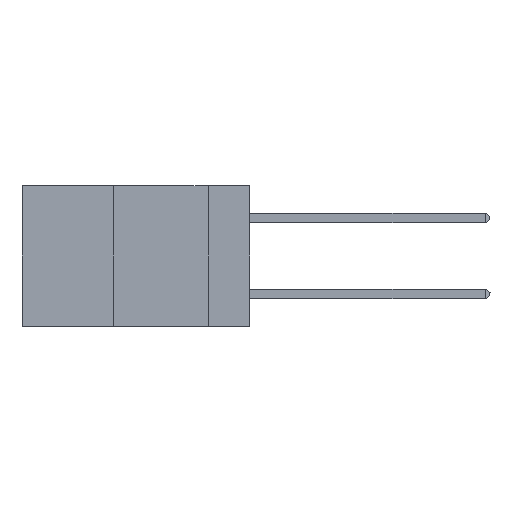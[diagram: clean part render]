
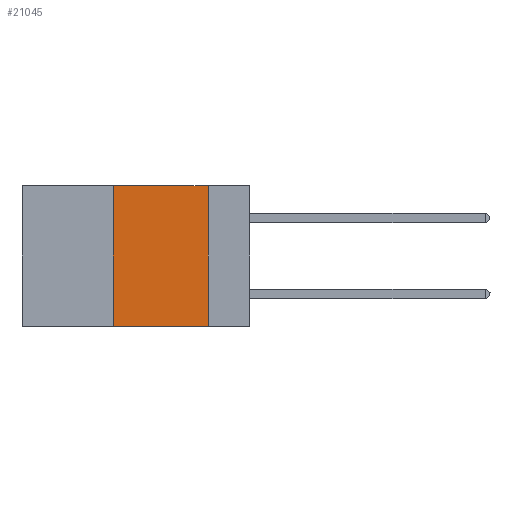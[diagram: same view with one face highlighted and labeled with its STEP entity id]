
A CAD part, left-side view. The second image highlights one B-rep face of the part: STEP entity #21045.
In plain terms, the highlighted planar face has unit normal (-1, 0, 0).
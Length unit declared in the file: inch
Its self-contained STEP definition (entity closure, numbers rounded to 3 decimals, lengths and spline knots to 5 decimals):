
#115 = LINE ( 'NONE', #12539, #3642 ) ;
#2055 = EDGE_CURVE ( 'NONE', #26909, #10300, #24432, .T. ) ;
#3494 = AXIS2_PLACEMENT_3D ( 'NONE', #9366, #14976, #14730 ) ;
#3642 = VECTOR ( 'NONE', #25003, 39.37008 ) ;
#3838 = ORIENTED_EDGE ( 'NONE', *, *, #23801, .F. ) ;
#5244 = EDGE_CURVE ( 'NONE', #10300, #28486, #23119, .T. ) ;
#5807 = DIRECTION ( 'NONE',  ( 0., 0., -1. ) ) ;
#8515 = CARTESIAN_POINT ( 'NONE',  ( 0., 0.6, -0.37 ) ) ;
#9284 = VECTOR ( 'NONE', #18669, 39.37008 ) ;
#9366 = CARTESIAN_POINT ( 'NONE',  ( 0., 0.6, 0. ) ) ;
#10300 = VERTEX_POINT ( 'NONE', #27777 ) ;
#10613 = CARTESIAN_POINT ( 'NONE',  ( 0., 0.11, 0. ) ) ;
#11392 = DIRECTION ( 'NONE',  ( 0., -1., 0. ) ) ;
#11901 = VERTEX_POINT ( 'NONE', #26102 ) ;
#11933 = ORIENTED_EDGE ( 'NONE', *, *, #2055, .F. ) ;
#12539 = CARTESIAN_POINT ( 'NONE',  ( 0., 0.36, 0. ) ) ;
#13627 = ORIENTED_EDGE ( 'NONE', *, *, #18059, .T. ) ;
#14730 = DIRECTION ( 'NONE',  ( 0., 0., -1. ) ) ;
#14976 = DIRECTION ( 'NONE',  ( 1., 0., 0. ) ) ;
#16281 = VECTOR ( 'NONE', #5807, 39.37008 ) ;
#17509 = ORIENTED_EDGE ( 'NONE', *, *, #5244, .F. ) ;
#17940 = CARTESIAN_POINT ( 'NONE',  ( 0., 0.36, 0. ) ) ;
#18059 = EDGE_CURVE ( 'NONE', #11901, #28486, #25909, .T. ) ;
#18669 = DIRECTION ( 'NONE',  ( 0., -1., 0. ) ) ;
#21045 = ADVANCED_FACE ( 'NONE', ( #28520 ), #24614, .F. ) ;
#22246 = CARTESIAN_POINT ( 'NONE',  ( 0., 0.6, 0. ) ) ;
#23119 = LINE ( 'NONE', #10613, #16281 ) ;
#23690 = CARTESIAN_POINT ( 'NONE',  ( 0., 0.11, -0.37 ) ) ;
#23801 = EDGE_CURVE ( 'NONE', #11901, #26909, #115, .T. ) ;
#24432 = LINE ( 'NONE', #22246, #9284 ) ;
#24614 = PLANE ( 'NONE',  #3494 ) ;
#25003 = DIRECTION ( 'NONE',  ( 0., 0., 1. ) ) ;
#25909 = LINE ( 'NONE', #8515, #31080 ) ;
#26102 = CARTESIAN_POINT ( 'NONE',  ( 0., 0.36, -0.37 ) ) ;
#26909 = VERTEX_POINT ( 'NONE', #17940 ) ;
#27383 = EDGE_LOOP ( 'NONE', ( #17509, #11933, #3838, #13627 ) ) ;
#27777 = CARTESIAN_POINT ( 'NONE',  ( 0., 0.11, 0. ) ) ;
#28486 = VERTEX_POINT ( 'NONE', #23690 ) ;
#28520 = FACE_OUTER_BOUND ( 'NONE', #27383, .T. ) ;
#31080 = VECTOR ( 'NONE', #11392, 39.37008 ) ;
